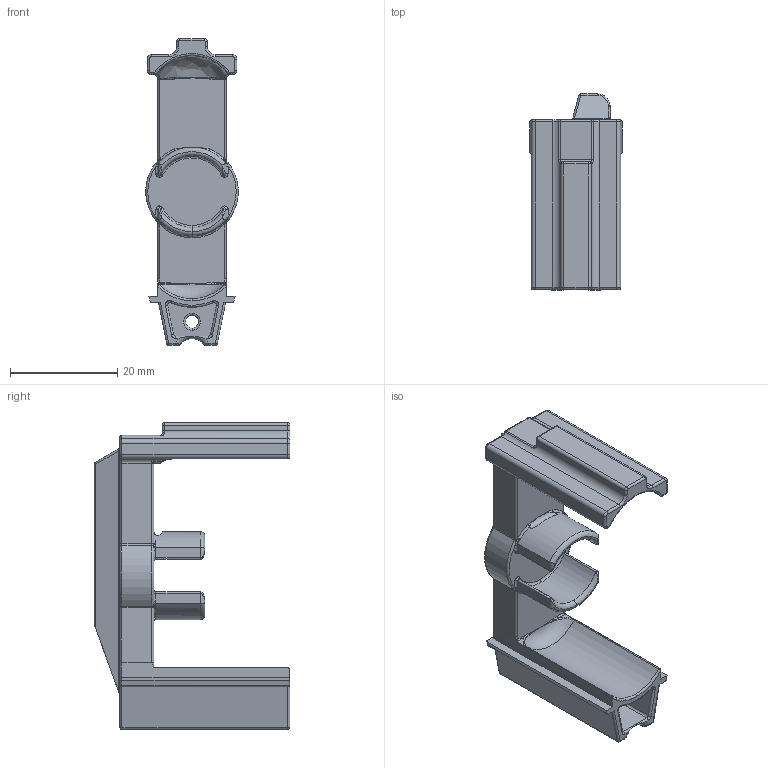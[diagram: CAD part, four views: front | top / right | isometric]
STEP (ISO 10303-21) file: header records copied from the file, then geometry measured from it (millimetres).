
FILE_DESCRIPTION(/* description */ ('STEP AP214'),/* implementation_level */ '2;1');
FILE_NAME(/* name */ 'Ivan''Ivan''s Standard Follower Without Brim.stp',/* time_stamp */ '2019-01-27T20:58:21-06:00',/* author */ ('johne'),/* organization */ (''),/* preprocessor_version */ 'ST-DEVELOPER v16.13',/* originating_system */ 'Autodesk Inventor 2018',/* authorisation */ '');
FILE_SCHEMA (('AUTOMOTIVE_DESIGN { 1 0 10303 214 3 1 1 }'));
Length unit declared in the file: millimetre
Products named in the file (1): DefDist_Cuomo_AR15_30_Mag_Follower
Bounding box: 17.22 x 36.53 x 57.28 mm (x, y, z)
Volume: 8963.7 mm3; surface area: 6533 mm2
Topology: 1 solids, 1 shells, 310 faces, 763 edges, 438 vertices
Faces by surface type: cylinder 118, bspline 67, torus 64, plane 52, sphere 9
Full cylindrical faces by diameter (mm): 2.388 x1
Entity records: 14275 total; most frequent: CARTESIAN_POINT 7324, ORIENTED_EDGE 1482, DIRECTION 1452, EDGE_CURVE 741, AXIS2_PLACEMENT_3D 597, VERTEX_POINT 436, EDGE_LOOP 311, CIRCLE 310
